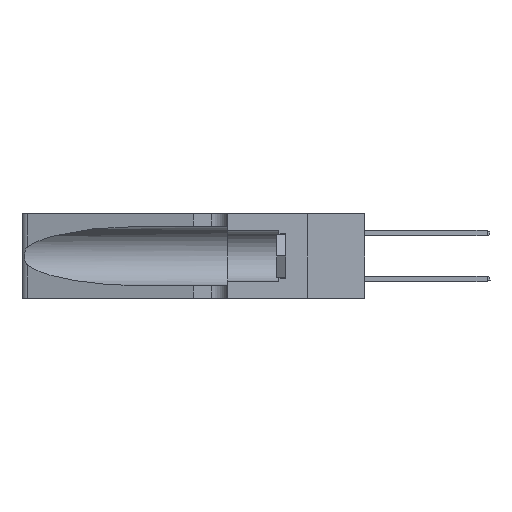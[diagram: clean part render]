
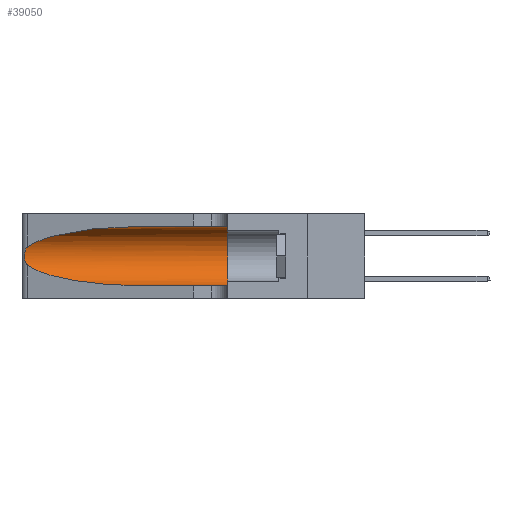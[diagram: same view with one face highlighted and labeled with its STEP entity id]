
A CAD part, left-side view. The second image highlights one B-rep face of the part: STEP entity #39050.
In plain terms, the highlighted cylindrical face has radius 3.308 mm (diameter 6.617 mm), a partial arc.
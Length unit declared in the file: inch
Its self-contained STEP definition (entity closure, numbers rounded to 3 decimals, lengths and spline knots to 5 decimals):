
#139 = VECTOR ( 'NONE', #30840, 39.37008 ) ;
#861 = VERTEX_POINT ( 'NONE', #19134 ) ;
#1136 = CARTESIAN_POINT ( 'NONE',  ( 0.25487, 1.22718, 0.22369 ) ) ;
#1355 = ORIENTED_EDGE ( 'NONE', *, *, #22667, .T. ) ;
#1428 = CARTESIAN_POINT ( 'NONE',  ( 0.26018, 1.23835, 0.19895 ) ) ;
#1500 = DIRECTION ( 'NONE',  ( 0., 1., 0. ) ) ;
#1575 = CARTESIAN_POINT ( 'NONE',  ( 0.26075, 1.23896, 0.178 ) ) ;
#2490 = CARTESIAN_POINT ( 'NONE',  ( 0.1305, 0.72297, 0.31525 ) ) ;
#2911 = CARTESIAN_POINT ( 'NONE',  ( 0.2373, 1.15595, 0.28018 ) ) ;
#3489 = VERTEX_POINT ( 'NONE', #7357 ) ;
#3491 = CARTESIAN_POINT ( 'NONE',  ( 0.1305, 0.35, 0.31525 ) ) ;
#3632 = CARTESIAN_POINT ( 'NONE',  ( 0.25487, 1.22718, 0.22369 ) ) ;
#4355 = CARTESIAN_POINT ( 'NONE',  ( 0.25854, 1.2359, 0.20912 ) ) ;
#4932 = CARTESIAN_POINT ( 'NONE',  ( 0.25487, 1.22718, 0.14631 ) ) ;
#6491 = LINE ( 'NONE', #31347, #32796 ) ;
#7357 = CARTESIAN_POINT ( 'NONE',  ( 0.1305, 0.72297, 0.31525 ) ) ;
#8860 = DIRECTION ( 'NONE',  ( 0., 0., -1. ) ) ;
#9003 = DIRECTION ( 'NONE',  ( 0., -1., 0. ) ) ;
#9515 = VERTEX_POINT ( 'NONE', #3632 ) ;
#10558 = ORIENTED_EDGE ( 'NONE', *, *, #31191, .F. ) ;
#10610 = AXIS2_PLACEMENT_3D ( 'NONE', #29296, #9003, #8860 ) ;
#10853 = CYLINDRICAL_SURFACE ( 'NONE', #10610, 0.13025 ) ;
#11189 = DIRECTION ( 'NONE',  ( 0., -1., 0. ) ) ;
#11288 = CARTESIAN_POINT ( 'NONE',  ( 0.25555, 1.22994, 0.2215 ) ) ;
#11664 = DIRECTION ( 'NONE',  ( 0., 0., 1. ) ) ;
#12651 = CARTESIAN_POINT ( 'NONE',  ( 0.18966, 0.96281, 0.31525 ) ) ;
#13864 = LINE ( 'NONE', #31437, #139 ) ;
#14187 = EDGE_LOOP ( 'NONE', ( #36727, #18585, #29616, #1355, #39848, #10558 ) ) ;
#15223 = CARTESIAN_POINT ( 'NONE',  ( 0.2373, 1.15595, 0.08982 ) ) ;
#15953 = EDGE_CURVE ( 'NONE', #3489, #9515, #38343, .T. ) ;
#16034 = CARTESIAN_POINT ( 'NONE',  ( 0.25487, 1.22718, 0.22369 ) ) ;
#17830 = EDGE_CURVE ( 'NONE', #9515, #43409, #42156, .T. ) ;
#18047 = CARTESIAN_POINT ( 'NONE',  ( 0.25787, 1.23484, 0.2124 ) ) ;
#18516 = AXIS2_PLACEMENT_3D ( 'NONE', #29009, #1500, #11664 ) ;
#18585 = ORIENTED_EDGE ( 'NONE', *, *, #17830, .T. ) ;
#19134 = CARTESIAN_POINT ( 'NONE',  ( 0.1305, 0.35, 0.05475 ) ) ;
#21332 = CARTESIAN_POINT ( 'NONE',  ( 0.25487, 1.22718, 0.14631 ) ) ;
#21402 = CARTESIAN_POINT ( 'NONE',  ( 0.1305, 0.72297, 0.05475 ) ) ;
#22267 = CARTESIAN_POINT ( 'NONE',  ( 0.18966, 0.96281, 0.05475 ) ) ;
#22432 = EDGE_CURVE ( 'NONE', #30026, #861, #31791, .T. ) ;
#22667 = EDGE_CURVE ( 'NONE', #38263, #861, #6491, .T. ) ;
#24507 = CARTESIAN_POINT ( 'NONE',  ( 0.25639, 1.23184, 0.21858 ) ) ;
#24840 =( BOUNDED_CURVE ( )  B_SPLINE_CURVE ( 3, ( #35815, #15223, #22267, #25490 ),
 .UNSPECIFIED., .F., .T. ) 
 B_SPLINE_CURVE_WITH_KNOTS ( ( 4, 4 ),
 ( 3.44316, 4.71239 ),
 .UNSPECIFIED. ) 
 CURVE ( )  GEOMETRIC_REPRESENTATION_ITEM ( )  RATIONAL_B_SPLINE_CURVE ( ( 1., 0.87, 0.87, 1. ) ) 
 REPRESENTATION_ITEM ( '' )  );
#25077 = CARTESIAN_POINT ( 'NONE',  ( 0.25639, 1.23186, 0.15144 ) ) ;
#25490 = CARTESIAN_POINT ( 'NONE',  ( 0.1305, 0.72297, 0.05475 ) ) ;
#25552 = FACE_OUTER_BOUND ( 'NONE', #14187, .T. ) ;
#28345 = CARTESIAN_POINT ( 'NONE',  ( 0.26017, 1.23833, 0.17102 ) ) ;
#29009 = CARTESIAN_POINT ( 'NONE',  ( 0.1305, 0.35, 0.185 ) ) ;
#29296 = CARTESIAN_POINT ( 'NONE',  ( 0.1305, 1.61858, 0.185 ) ) ;
#29616 = ORIENTED_EDGE ( 'NONE', *, *, #34120, .T. ) ;
#30026 = VERTEX_POINT ( 'NONE', #3491 ) ;
#30840 = DIRECTION ( 'NONE',  ( 0., -1., 0. ) ) ;
#31191 = EDGE_CURVE ( 'NONE', #3489, #30026, #13864, .T. ) ;
#31347 = CARTESIAN_POINT ( 'NONE',  ( 0.1305, 1.61858, 0.05475 ) ) ;
#31437 = CARTESIAN_POINT ( 'NONE',  ( 0.1305, 1.61858, 0.31525 ) ) ;
#31791 = CIRCLE ( 'NONE', #18516, 0.13025 ) ;
#32796 = VECTOR ( 'NONE', #11189, 39.37008 ) ;
#34120 = EDGE_CURVE ( 'NONE', #43409, #38263, #24840, .T. ) ;
#34831 = CARTESIAN_POINT ( 'NONE',  ( 0.26075, 1.23896, 0.19203 ) ) ;
#35122 = CARTESIAN_POINT ( 'NONE',  ( 0.25856, 1.23593, 0.16098 ) ) ;
#35815 = CARTESIAN_POINT ( 'NONE',  ( 0.25487, 1.22718, 0.14631 ) ) ;
#36727 = ORIENTED_EDGE ( 'NONE', *, *, #15953, .T. ) ;
#38057 = CARTESIAN_POINT ( 'NONE',  ( 0.25789, 1.23486, 0.15765 ) ) ;
#38263 = VERTEX_POINT ( 'NONE', #21402 ) ;
#38343 =( BOUNDED_CURVE ( )  B_SPLINE_CURVE ( 3, ( #2490, #12651, #2911, #16034 ),
 .UNSPECIFIED., .F., .F. ) 
 B_SPLINE_CURVE_WITH_KNOTS ( ( 4, 4 ),
 ( 1.5708, 2.84003 ),
 .UNSPECIFIED. ) 
 CURVE ( )  GEOMETRIC_REPRESENTATION_ITEM ( )  RATIONAL_B_SPLINE_CURVE ( ( 1., 0.87, 0.87, 1. ) ) 
 REPRESENTATION_ITEM ( '' )  );
#39050 = ADVANCED_FACE ( 'NONE', ( #25552 ), #10853, .F. ) ;
#39848 = ORIENTED_EDGE ( 'NONE', *, *, #22432, .F. ) ;
#41604 = CARTESIAN_POINT ( 'NONE',  ( 0.25555, 1.22993, 0.14849 ) ) ;
#42156 = B_SPLINE_CURVE_WITH_KNOTS ( 'NONE', 3,
 ( #1136, #11288, #24507, #18047, #4355, #1428, #34831, #1575, #28345, #35122, #38057, #25077, #41604, #4932 ),
 .UNSPECIFIED., .F., .F.,
 ( 4, 2, 2, 2, 2, 2, 4 ),
 ( 0., 0.00027, 0.00053, 0.00107, 0.0016, 0.00187, 0.00214 ),
 .UNSPECIFIED. ) ;
#43409 = VERTEX_POINT ( 'NONE', #21332 ) ;
